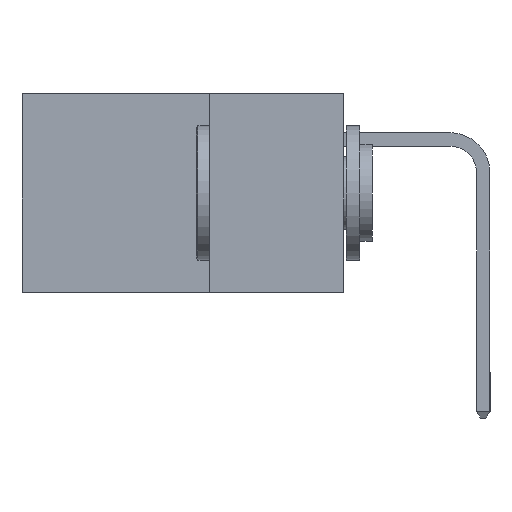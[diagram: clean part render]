
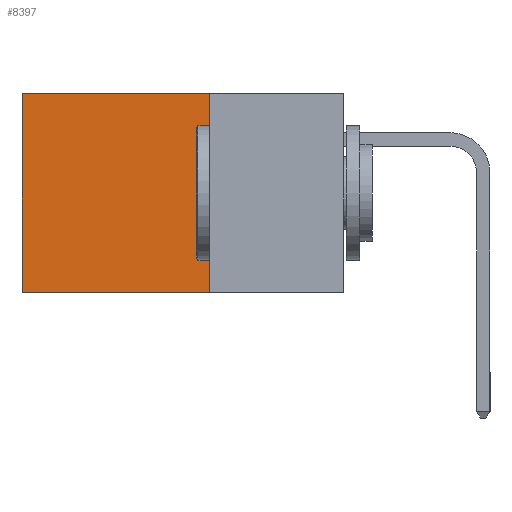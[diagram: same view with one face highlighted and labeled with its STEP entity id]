
A CAD part, left-side view. The second image highlights one B-rep face of the part: STEP entity #8397.
In plain terms, the highlighted planar face has unit normal (-1, 0, 0).
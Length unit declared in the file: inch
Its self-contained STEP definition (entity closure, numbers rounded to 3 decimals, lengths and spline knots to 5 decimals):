
#328 = EDGE_CURVE ( 'NONE', #18870, #20361, #7044, .T. ) ;
#1645 = CARTESIAN_POINT ( 'NONE',  ( 0.298, 0.25, 0. ) ) ;
#1865 = EDGE_CURVE ( 'NONE', #17554, #18870, #15876, .T. ) ;
#2056 = CARTESIAN_POINT ( 'NONE',  ( 0.298, 0.25, 0. ) ) ;
#2132 = CARTESIAN_POINT ( 'NONE',  ( 0.298, 0.25, 0. ) ) ;
#3136 = CARTESIAN_POINT ( 'NONE',  ( 0.298, 0.25, -0.37 ) ) ;
#3265 = CARTESIAN_POINT ( 'NONE',  ( 0.298, 0.6, -0.37 ) ) ;
#3400 = DIRECTION ( 'NONE',  ( 0., 0., -1. ) ) ;
#3872 = DIRECTION ( 'NONE',  ( 0., 0., -1. ) ) ;
#5352 = ORIENTED_EDGE ( 'NONE', *, *, #13377, .F. ) ;
#5896 = VECTOR ( 'NONE', #14391, 39.37008 ) ;
#6516 = ORIENTED_EDGE ( 'NONE', *, *, #14111, .F. ) ;
#7044 = LINE ( 'NONE', #16455, #20946 ) ;
#7609 = DIRECTION ( 'NONE',  ( 0., 1., 0. ) ) ;
#8397 = ADVANCED_FACE ( 'NONE', ( #13162 ), #16449, .F. ) ;
#9083 = AXIS2_PLACEMENT_3D ( 'NONE', #1645, #18503, #3872 ) ;
#9209 = CARTESIAN_POINT ( 'NONE',  ( 0.298, 0.25, 0. ) ) ;
#11223 = DIRECTION ( 'NONE',  ( 0., 0., -1. ) ) ;
#12071 = ORIENTED_EDGE ( 'NONE', *, *, #328, .T. ) ;
#13020 = VECTOR ( 'NONE', #7609, 39.37008 ) ;
#13162 = FACE_OUTER_BOUND ( 'NONE', #15347, .T. ) ;
#13377 = EDGE_CURVE ( 'NONE', #20639, #20361, #20320, .T. ) ;
#14095 = CARTESIAN_POINT ( 'NONE',  ( 0.298, 0.6, 0. ) ) ;
#14111 = EDGE_CURVE ( 'NONE', #17554, #20639, #17350, .T. ) ;
#14391 = DIRECTION ( 'NONE',  ( 0., 1., 0. ) ) ;
#15347 = EDGE_LOOP ( 'NONE', ( #12071, #5352, #6516, #18672 ) ) ;
#15876 = LINE ( 'NONE', #2132, #13020 ) ;
#16449 = PLANE ( 'NONE',  #9083 ) ;
#16455 = CARTESIAN_POINT ( 'NONE',  ( 0.298, 0.6, 0. ) ) ;
#17350 = LINE ( 'NONE', #9209, #23766 ) ;
#17554 = VERTEX_POINT ( 'NONE', #2056 ) ;
#18503 = DIRECTION ( 'NONE',  ( 1., 0., 0. ) ) ;
#18672 = ORIENTED_EDGE ( 'NONE', *, *, #1865, .T. ) ;
#18870 = VERTEX_POINT ( 'NONE', #14095 ) ;
#20320 = LINE ( 'NONE', #3136, #5896 ) ;
#20361 = VERTEX_POINT ( 'NONE', #3265 ) ;
#20639 = VERTEX_POINT ( 'NONE', #20686 ) ;
#20686 = CARTESIAN_POINT ( 'NONE',  ( 0.298, 0.25, -0.37 ) ) ;
#20946 = VECTOR ( 'NONE', #3400, 39.37008 ) ;
#23766 = VECTOR ( 'NONE', #11223, 39.37008 ) ;
